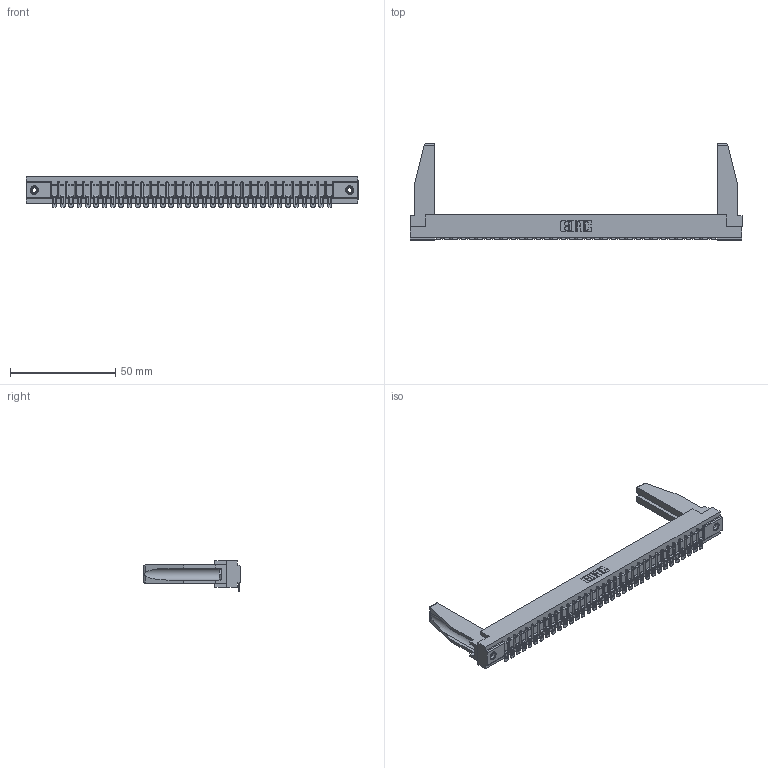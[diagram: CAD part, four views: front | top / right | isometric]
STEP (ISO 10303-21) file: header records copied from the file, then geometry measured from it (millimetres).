
FILE_DESCRIPTION (( 'STEP AP203' ), '1' );
FILE_NAME ('357-034-554-178.STEP', '2019-09-17T05:39:15', ( '' ), ( '' ), 'SwSTEP 2.0', 'SolidWorks 2016', '' );
FILE_SCHEMA (( 'CONFIG_CONTROL_DESIGN' ));
Length unit declared in the file: inch
Products named in the file (5): 307 Part_.156 Dia Mounting Holes; 307-290-002_554; 307-220-078; 345-250-001_345-250-001-102; 357-034-554-178
Assembly tree (39 placements, depth 2):
  357-034-554-178
    307 Part_.156 Dia Mounting Holes
    307-290-002_554  x34
    307-220-078  x2
    345-250-001_345-250-001-102  x2
Bounding box: 157.73 x 45.72 x 14.52 mm (x, y, z)
Volume: 20825.5 mm3; surface area: 24945.1 mm2
Topology: 39 solids, 39 shells, 3037 faces, 9255 edges, 6066 vertices
Faces by surface type: plane 1718, cylinder 1233, sphere 70, cone 12, torus 4
Entity records: 33538 total; most frequent: CARTESIAN_POINT 5656, ORIENTED_EDGE 5602, DIRECTION 5461, EDGE_CURVE 2801, VECTOR 2139, LINE 2139, VERTEX_POINT 1814, AXIS2_PLACEMENT_3D 1661
